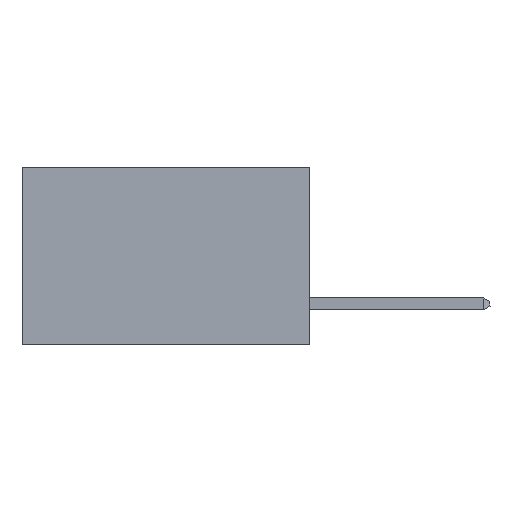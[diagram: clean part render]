
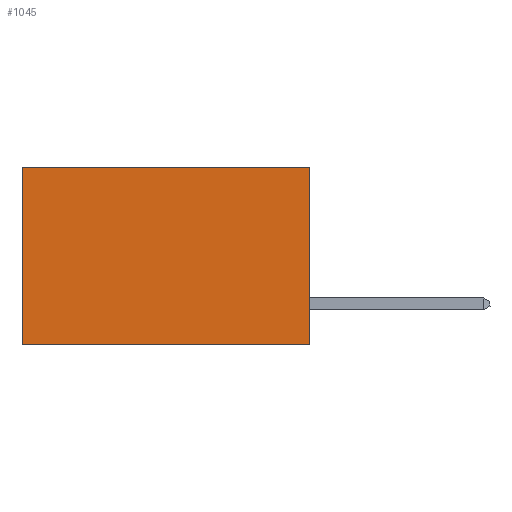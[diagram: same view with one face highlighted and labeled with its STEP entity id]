
A CAD part, left-side view. The second image highlights one B-rep face of the part: STEP entity #1045.
In plain terms, the highlighted planar face has unit normal (-1, 0, 0).
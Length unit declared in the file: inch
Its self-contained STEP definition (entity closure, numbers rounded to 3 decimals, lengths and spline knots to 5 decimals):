
#156 = EDGE_CURVE ( 'NONE', #13735, #3881, #14278, .T. ) ;
#365 = DIRECTION ( 'NONE',  ( 0., 0., -1. ) ) ;
#1045 = ADVANCED_FACE ( 'NONE', ( #10008 ), #8111, .F. ) ;
#1299 = CARTESIAN_POINT ( 'NONE',  ( 0.2875, 0.6, 0. ) ) ;
#1719 = CARTESIAN_POINT ( 'NONE',  ( 0.2875, 0., 0. ) ) ;
#2282 = VERTEX_POINT ( 'NONE', #1719 ) ;
#3835 = CARTESIAN_POINT ( 'NONE',  ( 0.2875, 0.6, 0. ) ) ;
#3881 = VERTEX_POINT ( 'NONE', #5252 ) ;
#4333 = VECTOR ( 'NONE', #365, 39.37008 ) ;
#4462 = ORIENTED_EDGE ( 'NONE', *, *, #10678, .T. ) ;
#4531 = CARTESIAN_POINT ( 'NONE',  ( 0.2875, 0., 0. ) ) ;
#5222 = CARTESIAN_POINT ( 'NONE',  ( 0.2875, 0., 0. ) ) ;
#5252 = CARTESIAN_POINT ( 'NONE',  ( 0.2875, 0.6, -0.37 ) ) ;
#5767 = DIRECTION ( 'NONE',  ( 0., 1., 0. ) ) ;
#5902 = ORIENTED_EDGE ( 'NONE', *, *, #7425, .F. ) ;
#6122 = AXIS2_PLACEMENT_3D ( 'NONE', #6804, #10451, #11611 ) ;
#6449 = CARTESIAN_POINT ( 'NONE',  ( 0.2875, 0., -0.37 ) ) ;
#6479 = EDGE_LOOP ( 'NONE', ( #4462, #14568, #5902, #12536 ) ) ;
#6804 = CARTESIAN_POINT ( 'NONE',  ( 0.2875, 0., 0. ) ) ;
#7425 = EDGE_CURVE ( 'NONE', #2282, #13735, #11892, .T. ) ;
#7641 = LINE ( 'NONE', #3835, #4333 ) ;
#8111 = PLANE ( 'NONE',  #6122 ) ;
#8595 = VECTOR ( 'NONE', #5767, 39.37008 ) ;
#8770 = VECTOR ( 'NONE', #9845, 39.37008 ) ;
#9002 = DIRECTION ( 'NONE',  ( 0., 1., 0. ) ) ;
#9536 = VERTEX_POINT ( 'NONE', #1299 ) ;
#9678 = VECTOR ( 'NONE', #9002, 39.37008 ) ;
#9845 = DIRECTION ( 'NONE',  ( 0., 0., -1. ) ) ;
#10008 = FACE_OUTER_BOUND ( 'NONE', #6479, .T. ) ;
#10451 = DIRECTION ( 'NONE',  ( 1., 0., 0. ) ) ;
#10678 = EDGE_CURVE ( 'NONE', #9536, #3881, #7641, .T. ) ;
#11040 = EDGE_CURVE ( 'NONE', #2282, #9536, #14109, .T. ) ;
#11611 = DIRECTION ( 'NONE',  ( 0., 0., -1. ) ) ;
#11854 = CARTESIAN_POINT ( 'NONE',  ( 0.2875, 0., -0.37 ) ) ;
#11892 = LINE ( 'NONE', #5222, #8770 ) ;
#12536 = ORIENTED_EDGE ( 'NONE', *, *, #11040, .T. ) ;
#13735 = VERTEX_POINT ( 'NONE', #11854 ) ;
#14109 = LINE ( 'NONE', #4531, #8595 ) ;
#14278 = LINE ( 'NONE', #6449, #9678 ) ;
#14568 = ORIENTED_EDGE ( 'NONE', *, *, #156, .F. ) ;
